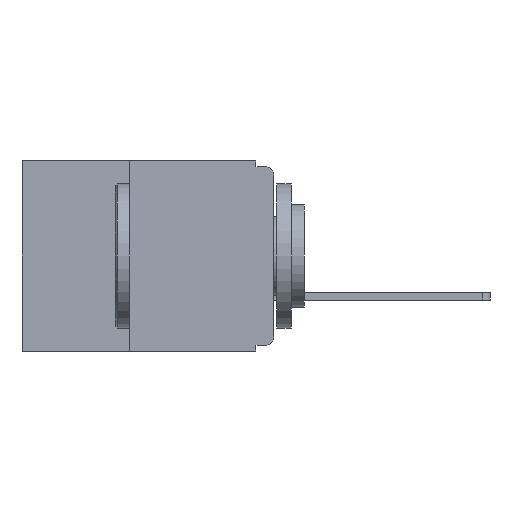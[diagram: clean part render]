
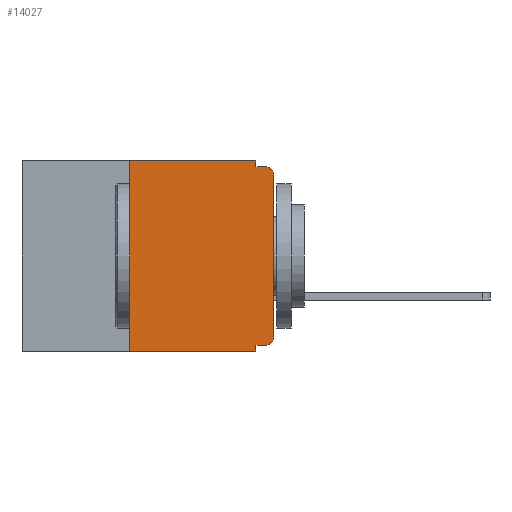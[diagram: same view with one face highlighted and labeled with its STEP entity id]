
A CAD part, left-side view. The second image highlights one B-rep face of the part: STEP entity #14027.
In plain terms, the highlighted planar face has unit normal (-1, 0, 0).
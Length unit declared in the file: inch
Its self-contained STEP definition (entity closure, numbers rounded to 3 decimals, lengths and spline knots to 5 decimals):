
#844 = CARTESIAN_POINT ( 'NONE',  ( 0., 0., -0.01 ) ) ;
#1061 = LINE ( 'NONE', #9861, #24912 ) ;
#1524 = VECTOR ( 'NONE', #12173, 39.37008 ) ;
#1842 = ORIENTED_EDGE ( 'NONE', *, *, #15546, .F. ) ;
#2863 = CARTESIAN_POINT ( 'NONE',  ( 0., 0., 0. ) ) ;
#3667 = LINE ( 'NONE', #13752, #15559 ) ;
#4065 = LINE ( 'NONE', #18270, #27772 ) ;
#4453 = ORIENTED_EDGE ( 'NONE', *, *, #15872, .T. ) ;
#4592 = LINE ( 'NONE', #2863, #22847 ) ;
#4880 = CARTESIAN_POINT ( 'NONE',  ( 0., 0.25, -0.33 ) ) ;
#5183 = CARTESIAN_POINT ( 'NONE',  ( 0., 0.25, 0. ) ) ;
#5221 = AXIS2_PLACEMENT_3D ( 'NONE', #6109, #22782, #8548 ) ;
#5830 = VERTEX_POINT ( 'NONE', #13987 ) ;
#6109 = CARTESIAN_POINT ( 'NONE',  ( 0., 0.015, -0.025 ) ) ;
#6403 = CARTESIAN_POINT ( 'NONE',  ( 0., 0.031, -0.01 ) ) ;
#6729 = PLANE ( 'NONE',  #9339 ) ;
#7851 = CIRCLE ( 'NONE', #5221, 0.015 ) ;
#8000 = VECTOR ( 'NONE', #13407, 39.37008 ) ;
#8055 = FACE_OUTER_BOUND ( 'NONE', #20611, .T. ) ;
#8188 = CARTESIAN_POINT ( 'NONE',  ( 0., 0.015, -0.305 ) ) ;
#8548 = DIRECTION ( 'NONE',  ( 0., 0., -1. ) ) ;
#8555 = VERTEX_POINT ( 'NONE', #6403 ) ;
#8954 = EDGE_CURVE ( 'NONE', #11592, #21176, #1061, .T. ) ;
#9270 = EDGE_CURVE ( 'NONE', #29025, #8555, #4065, .T. ) ;
#9339 = AXIS2_PLACEMENT_3D ( 'NONE', #18607, #25736, #11535 ) ;
#9528 = CIRCLE ( 'NONE', #13779, 0.015 ) ;
#9861 = CARTESIAN_POINT ( 'NONE',  ( 0., 0.437, -0.33 ) ) ;
#10260 = ORIENTED_EDGE ( 'NONE', *, *, #30682, .F. ) ;
#10581 = DIRECTION ( 'NONE',  ( 0., 0., -1. ) ) ;
#11535 = DIRECTION ( 'NONE',  ( 0., 0., -1. ) ) ;
#11592 = VERTEX_POINT ( 'NONE', #25185 ) ;
#11856 = CARTESIAN_POINT ( 'NONE',  ( 0., 0.031, 0. ) ) ;
#12095 = ORIENTED_EDGE ( 'NONE', *, *, #17799, .T. ) ;
#12173 = DIRECTION ( 'NONE',  ( 0., 1., 0. ) ) ;
#12776 = DIRECTION ( 'NONE',  ( 0., -1., 0. ) ) ;
#13407 = DIRECTION ( 'NONE',  ( 0., -1., 0. ) ) ;
#13752 = CARTESIAN_POINT ( 'NONE',  ( 0., 0.031, -0.33 ) ) ;
#13779 = AXIS2_PLACEMENT_3D ( 'NONE', #8188, #24796, #10581 ) ;
#13987 = CARTESIAN_POINT ( 'NONE',  ( 0., 0., -0.305 ) ) ;
#14027 = ADVANCED_FACE ( 'NONE', ( #8055 ), #6729, .F. ) ;
#14683 = EDGE_CURVE ( 'NONE', #11592, #26190, #21036, .T. ) ;
#14828 = ORIENTED_EDGE ( 'NONE', *, *, #29104, .F. ) ;
#15546 = EDGE_CURVE ( 'NONE', #26190, #29025, #26889, .T. ) ;
#15559 = VECTOR ( 'NONE', #23289, 39.37008 ) ;
#15627 = VERTEX_POINT ( 'NONE', #16071 ) ;
#15716 = LINE ( 'NONE', #844, #21322 ) ;
#15872 = EDGE_CURVE ( 'NONE', #5830, #17350, #4592, .T. ) ;
#16071 = CARTESIAN_POINT ( 'NONE',  ( 0., 0.031, -0.32 ) ) ;
#16285 = ORIENTED_EDGE ( 'NONE', *, *, #14683, .F. ) ;
#16756 = DIRECTION ( 'NONE',  ( 0., 0., 1. ) ) ;
#17107 = DIRECTION ( 'NONE',  ( 0., 0., 1. ) ) ;
#17350 = VERTEX_POINT ( 'NONE', #22443 ) ;
#17799 = EDGE_CURVE ( 'NONE', #17350, #21539, #7851, .T. ) ;
#18270 = CARTESIAN_POINT ( 'NONE',  ( 0., 0.031, 0. ) ) ;
#18607 = CARTESIAN_POINT ( 'NONE',  ( 0., 0.437, 0. ) ) ;
#19808 = LINE ( 'NONE', #26326, #1524 ) ;
#20281 = VECTOR ( 'NONE', #16756, 39.37008 ) ;
#20611 = EDGE_LOOP ( 'NONE', ( #4453, #12095, #22068, #23240, #1842, #16285, #21038, #10260, #14828, #21049 ) ) ;
#21036 = LINE ( 'NONE', #4880, #20281 ) ;
#21038 = ORIENTED_EDGE ( 'NONE', *, *, #8954, .T. ) ;
#21049 = ORIENTED_EDGE ( 'NONE', *, *, #26944, .T. ) ;
#21176 = VERTEX_POINT ( 'NONE', #24567 ) ;
#21322 = VECTOR ( 'NONE', #12776, 39.37008 ) ;
#21539 = VERTEX_POINT ( 'NONE', #28681 ) ;
#22068 = ORIENTED_EDGE ( 'NONE', *, *, #28629, .F. ) ;
#22443 = CARTESIAN_POINT ( 'NONE',  ( 0., 0., -0.025 ) ) ;
#22782 = DIRECTION ( 'NONE',  ( -1., 0., 0. ) ) ;
#22847 = VECTOR ( 'NONE', #17107, 39.37008 ) ;
#22856 = CARTESIAN_POINT ( 'NONE',  ( 0., 0.437, 0. ) ) ;
#23240 = ORIENTED_EDGE ( 'NONE', *, *, #9270, .F. ) ;
#23289 = DIRECTION ( 'NONE',  ( 0., 0., -1. ) ) ;
#24172 = DIRECTION ( 'NONE',  ( 0., -1., 0. ) ) ;
#24567 = CARTESIAN_POINT ( 'NONE',  ( 0., 0.031, -0.33 ) ) ;
#24796 = DIRECTION ( 'NONE',  ( -1., 0., 0. ) ) ;
#24912 = VECTOR ( 'NONE', #24172, 39.37008 ) ;
#25185 = CARTESIAN_POINT ( 'NONE',  ( 0., 0.25, -0.33 ) ) ;
#25666 = CARTESIAN_POINT ( 'NONE',  ( 0., 0.015, -0.32 ) ) ;
#25736 = DIRECTION ( 'NONE',  ( 1., 0., 0. ) ) ;
#25968 = VERTEX_POINT ( 'NONE', #25666 ) ;
#26190 = VERTEX_POINT ( 'NONE', #5183 ) ;
#26326 = CARTESIAN_POINT ( 'NONE',  ( 0., 0., -0.32 ) ) ;
#26889 = LINE ( 'NONE', #22856, #8000 ) ;
#26944 = EDGE_CURVE ( 'NONE', #25968, #5830, #9528, .T. ) ;
#27719 = DIRECTION ( 'NONE',  ( 0., 0., -1. ) ) ;
#27772 = VECTOR ( 'NONE', #27719, 39.37008 ) ;
#28629 = EDGE_CURVE ( 'NONE', #8555, #21539, #15716, .T. ) ;
#28681 = CARTESIAN_POINT ( 'NONE',  ( 0., 0.015, -0.01 ) ) ;
#29025 = VERTEX_POINT ( 'NONE', #11856 ) ;
#29104 = EDGE_CURVE ( 'NONE', #25968, #15627, #19808, .T. ) ;
#30682 = EDGE_CURVE ( 'NONE', #15627, #21176, #3667, .T. ) ;
